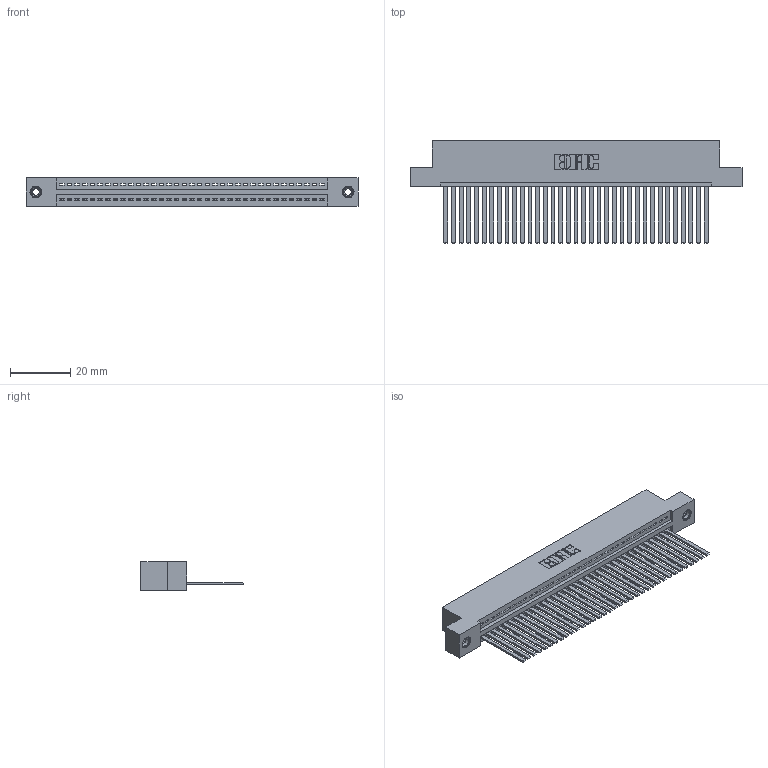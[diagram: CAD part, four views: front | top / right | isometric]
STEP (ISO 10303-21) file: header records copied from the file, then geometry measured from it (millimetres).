
FILE_DESCRIPTION (( 'STEP AP203' ), '1' );
FILE_NAME ('345-035-544-108.STEP', '2019-10-07T21:37:08', ( '' ), ( '' ), 'SwSTEP 2.0', 'SolidWorks 2016', '' );
FILE_SCHEMA (( 'CONFIG_CONTROL_DESIGN' ));
Length unit declared in the file: inch
Products named in the file (4): 345-035-544-108; 345 Part_Flush Mounting Lugs - 0.156 Dia-TI; 345-250-001_345-250-003-102; 345-292-001_345-293-144
Assembly tree (38 placements, depth 2):
  345-035-544-108
    345 Part_Flush Mounting Lugs - 0.156 Dia-TI
    345-292-001_345-293-144  x35
    345-250-001_345-250-003-102  x2
Bounding box: 110.11 x 33.96 x 9.4 mm (x, y, z)
Volume: 10799.7 mm3; surface area: 15492.8 mm2
Topology: 38 solids, 38 shells, 2006 faces, 6007 edges, 3950 vertices
Faces by surface type: plane 1372, cylinder 618, cone 12, torus 4
Entity records: 28286 total; most frequent: CARTESIAN_POINT 4880, ORIENTED_EDGE 4842, DIRECTION 4297, EDGE_CURVE 2421, VECTOR 2133, LINE 2133, VERTEX_POINT 1608, AXIS2_PLACEMENT_3D 1082
